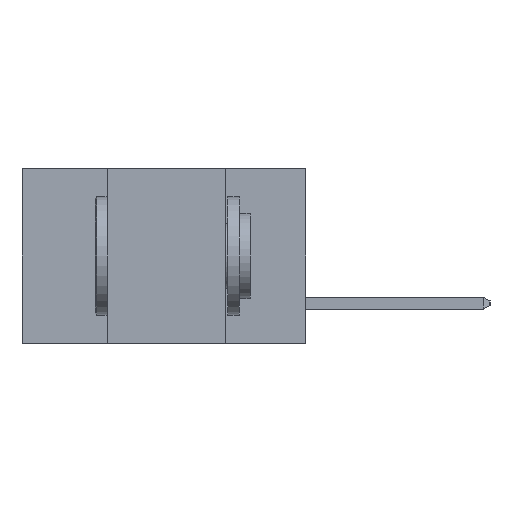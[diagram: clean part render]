
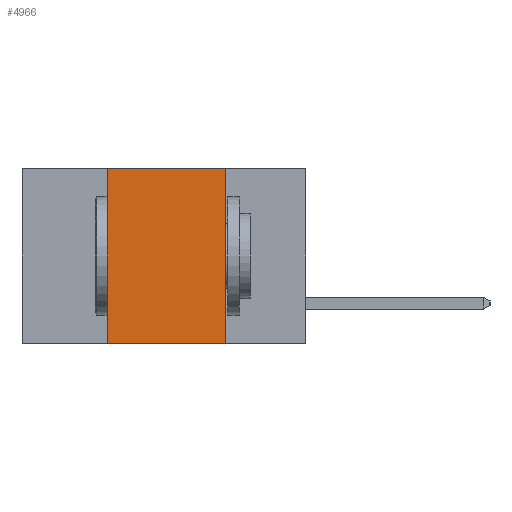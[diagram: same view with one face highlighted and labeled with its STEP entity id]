
A CAD part, left-side view. The second image highlights one B-rep face of the part: STEP entity #4966.
In plain terms, the highlighted planar face has unit normal (-1, 0, 0).
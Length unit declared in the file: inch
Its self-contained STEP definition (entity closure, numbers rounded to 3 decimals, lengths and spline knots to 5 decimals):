
#65 = LINE ( 'NONE', #3527, #3450 ) ;
#186 = EDGE_CURVE ( 'NONE', #6399, #1214, #65, .T. ) ;
#259 = VECTOR ( 'NONE', #2848, 39.37008 ) ;
#958 = DIRECTION ( 'NONE',  ( 0., -1., 0. ) ) ;
#976 = CARTESIAN_POINT ( 'NONE',  ( 0., 0.6, -0.37 ) ) ;
#1214 = VERTEX_POINT ( 'NONE', #7964 ) ;
#1288 = ORIENTED_EDGE ( 'NONE', *, *, #186, .F. ) ;
#1371 = DIRECTION ( 'NONE',  ( 0., -1., 0. ) ) ;
#1514 = ORIENTED_EDGE ( 'NONE', *, *, #3448, .F. ) ;
#1543 = CARTESIAN_POINT ( 'NONE',  ( 0., 0.6, 0. ) ) ;
#1639 = ORIENTED_EDGE ( 'NONE', *, *, #8621, .F. ) ;
#1931 = CARTESIAN_POINT ( 'NONE',  ( 0., 0.42, 0. ) ) ;
#2160 = CARTESIAN_POINT ( 'NONE',  ( 0., 0.42, -0.37 ) ) ;
#2520 = VECTOR ( 'NONE', #958, 39.37008 ) ;
#2848 = DIRECTION ( 'NONE',  ( 0., 0., 1. ) ) ;
#2869 = DIRECTION ( 'NONE',  ( 0., 0., -1. ) ) ;
#2878 = DIRECTION ( 'NONE',  ( 1., 0., 0. ) ) ;
#2898 = CARTESIAN_POINT ( 'NONE',  ( 0., 0.6, 0. ) ) ;
#2943 = LINE ( 'NONE', #1543, #4600 ) ;
#2955 = PLANE ( 'NONE',  #4098 ) ;
#3448 = EDGE_CURVE ( 'NONE', #7782, #6399, #2943, .T. ) ;
#3450 = VECTOR ( 'NONE', #5648, 39.37008 ) ;
#3527 = CARTESIAN_POINT ( 'NONE',  ( 0., 0.17, -0.37 ) ) ;
#3930 = LINE ( 'NONE', #976, #2520 ) ;
#4098 = AXIS2_PLACEMENT_3D ( 'NONE', #2898, #2878, #2869 ) ;
#4214 = EDGE_CURVE ( 'NONE', #8684, #1214, #3930, .T. ) ;
#4600 = VECTOR ( 'NONE', #1371, 39.37008 ) ;
#4966 = ADVANCED_FACE ( 'NONE', ( #9140 ), #2955, .F. ) ;
#5494 = CARTESIAN_POINT ( 'NONE',  ( 0., 0.17, 0. ) ) ;
#5530 = EDGE_LOOP ( 'NONE', ( #1288, #1514, #1639, #7003 ) ) ;
#5648 = DIRECTION ( 'NONE',  ( 0., 0., -1. ) ) ;
#6399 = VERTEX_POINT ( 'NONE', #5494 ) ;
#7003 = ORIENTED_EDGE ( 'NONE', *, *, #4214, .T. ) ;
#7192 = CARTESIAN_POINT ( 'NONE',  ( 0., 0.42, -0.37 ) ) ;
#7782 = VERTEX_POINT ( 'NONE', #1931 ) ;
#7853 = LINE ( 'NONE', #2160, #259 ) ;
#7964 = CARTESIAN_POINT ( 'NONE',  ( 0., 0.17, -0.37 ) ) ;
#8621 = EDGE_CURVE ( 'NONE', #8684, #7782, #7853, .T. ) ;
#8684 = VERTEX_POINT ( 'NONE', #7192 ) ;
#9140 = FACE_OUTER_BOUND ( 'NONE', #5530, .T. ) ;
